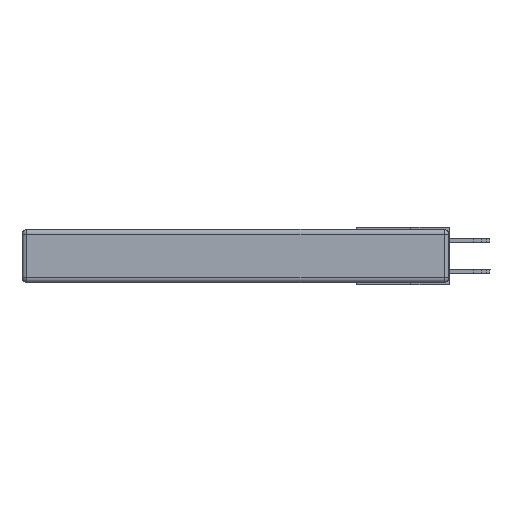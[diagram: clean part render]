
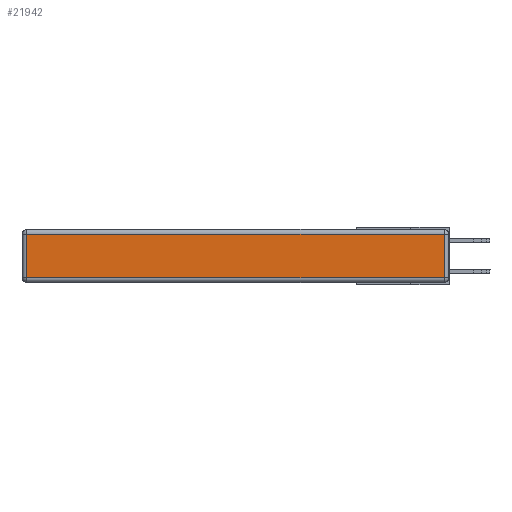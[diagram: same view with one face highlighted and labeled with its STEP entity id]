
A CAD part, left-side view. The second image highlights one B-rep face of the part: STEP entity #21942.
In plain terms, the highlighted planar face has unit normal (-1, 0, 0).
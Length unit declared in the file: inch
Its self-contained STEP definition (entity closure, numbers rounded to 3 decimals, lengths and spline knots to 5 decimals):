
#1493 = CARTESIAN_POINT ( 'NONE',  ( 0., 0., -0.343 ) ) ;
#1607 = LINE ( 'NONE', #21554, #6956 ) ;
#1627 = FACE_OUTER_BOUND ( 'NONE', #8076, .T. ) ;
#2547 = EDGE_CURVE ( 'NONE', #13779, #17481, #7665, .T. ) ;
#3241 = DIRECTION ( 'NONE',  ( 0., 0., 1. ) ) ;
#3570 = VERTEX_POINT ( 'NONE', #21053 ) ;
#4449 = EDGE_CURVE ( 'NONE', #17481, #3570, #9225, .T. ) ;
#4677 = CARTESIAN_POINT ( 'NONE',  ( 0., 0.03, -0.343 ) ) ;
#5006 = EDGE_CURVE ( 'NONE', #11075, #13779, #1607, .T. ) ;
#5372 = ORIENTED_EDGE ( 'NONE', *, *, #4449, .T. ) ;
#6575 = VECTOR ( 'NONE', #16755, 39.37008 ) ;
#6909 = ORIENTED_EDGE ( 'NONE', *, *, #5006, .T. ) ;
#6956 = VECTOR ( 'NONE', #21320, 39.37008 ) ;
#7665 = LINE ( 'NONE', #13095, #6575 ) ;
#8076 = EDGE_LOOP ( 'NONE', ( #20731, #5372, #16338, #6909 ) ) ;
#9225 = LINE ( 'NONE', #4677, #9486 ) ;
#9486 = VECTOR ( 'NONE', #22127, 39.37008 ) ;
#10018 = LINE ( 'NONE', #18866, #10538 ) ;
#10538 = VECTOR ( 'NONE', #22306, 39.37008 ) ;
#11075 = VERTEX_POINT ( 'NONE', #11126 ) ;
#11126 = CARTESIAN_POINT ( 'NONE',  ( 0., 2.72, -0.03 ) ) ;
#11771 = EDGE_CURVE ( 'NONE', #3570, #11075, #10018, .T. ) ;
#13095 = CARTESIAN_POINT ( 'NONE',  ( 0., 0., -0.313 ) ) ;
#13626 = DIRECTION ( 'NONE',  ( -1., 0., 0. ) ) ;
#13628 = CARTESIAN_POINT ( 'NONE',  ( 0., 0.03, -0.313 ) ) ;
#13779 = VERTEX_POINT ( 'NONE', #15140 ) ;
#15140 = CARTESIAN_POINT ( 'NONE',  ( 0., 2.72, -0.313 ) ) ;
#15265 = PLANE ( 'NONE',  #19764 ) ;
#16338 = ORIENTED_EDGE ( 'NONE', *, *, #11771, .T. ) ;
#16755 = DIRECTION ( 'NONE',  ( 0., -1., 0. ) ) ;
#17481 = VERTEX_POINT ( 'NONE', #13628 ) ;
#18866 = CARTESIAN_POINT ( 'NONE',  ( 0., 2.75, -0.03 ) ) ;
#19764 = AXIS2_PLACEMENT_3D ( 'NONE', #1493, #13626, #3241 ) ;
#20731 = ORIENTED_EDGE ( 'NONE', *, *, #2547, .T. ) ;
#21053 = CARTESIAN_POINT ( 'NONE',  ( 0., 0.03, -0.03 ) ) ;
#21320 = DIRECTION ( 'NONE',  ( 0., 0., -1. ) ) ;
#21554 = CARTESIAN_POINT ( 'NONE',  ( 0., 2.72, -0.343 ) ) ;
#21942 = ADVANCED_FACE ( 'NONE', ( #1627 ), #15265, .T. ) ;
#22127 = DIRECTION ( 'NONE',  ( 0., 0., 1. ) ) ;
#22306 = DIRECTION ( 'NONE',  ( 0., 1., 0. ) ) ;
